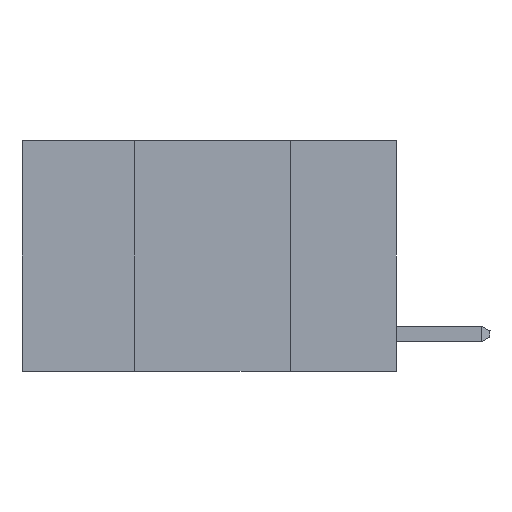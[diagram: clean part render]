
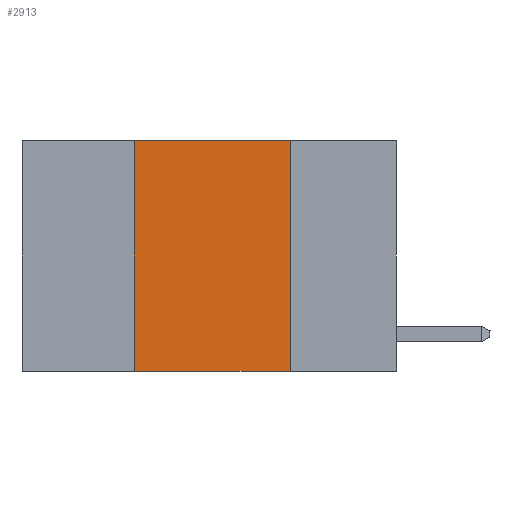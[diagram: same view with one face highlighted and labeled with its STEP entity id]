
A CAD part, left-side view. The second image highlights one B-rep face of the part: STEP entity #2913.
In plain terms, the highlighted planar face has unit normal (-1, 0, 0).
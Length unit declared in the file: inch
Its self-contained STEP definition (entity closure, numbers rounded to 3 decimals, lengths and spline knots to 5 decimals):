
#438 = CARTESIAN_POINT ( 'NONE',  ( 0., 0.17, 0. ) ) ;
#893 = VECTOR ( 'NONE', #7724, 39.37008 ) ;
#957 = LINE ( 'NONE', #9798, #1074 ) ;
#1074 = VECTOR ( 'NONE', #5204, 39.37008 ) ;
#2290 = DIRECTION ( 'NONE',  ( 0., -1., 0. ) ) ;
#2453 = CARTESIAN_POINT ( 'NONE',  ( 0., 0.17, 0. ) ) ;
#2671 = CARTESIAN_POINT ( 'NONE',  ( 0., 0.6, -0.37 ) ) ;
#2913 = ADVANCED_FACE ( 'NONE', ( #14982 ), #18160, .F. ) ;
#2950 = ORIENTED_EDGE ( 'NONE', *, *, #8047, .F. ) ;
#4691 = AXIS2_PLACEMENT_3D ( 'NONE', #7805, #10606, #16529 ) ;
#5204 = DIRECTION ( 'NONE',  ( 0., 0., 1. ) ) ;
#6109 = EDGE_LOOP ( 'NONE', ( #2950, #14230, #10822, #17636 ) ) ;
#6267 = CARTESIAN_POINT ( 'NONE',  ( 0., 0.42, 0. ) ) ;
#6475 = VERTEX_POINT ( 'NONE', #2453 ) ;
#7020 = EDGE_CURVE ( 'NONE', #18654, #6475, #7302, .T. ) ;
#7302 = LINE ( 'NONE', #9135, #10634 ) ;
#7724 = DIRECTION ( 'NONE',  ( 0., 0., -1. ) ) ;
#7805 = CARTESIAN_POINT ( 'NONE',  ( 0., 0.6, 0. ) ) ;
#8047 = EDGE_CURVE ( 'NONE', #6475, #12173, #13732, .T. ) ;
#9135 = CARTESIAN_POINT ( 'NONE',  ( 0., 0.6, 0. ) ) ;
#9798 = CARTESIAN_POINT ( 'NONE',  ( 0., 0.42, 0. ) ) ;
#10606 = DIRECTION ( 'NONE',  ( 1., 0., 0. ) ) ;
#10634 = VECTOR ( 'NONE', #14945, 39.37008 ) ;
#10822 = ORIENTED_EDGE ( 'NONE', *, *, #12796, .F. ) ;
#12173 = VERTEX_POINT ( 'NONE', #17082 ) ;
#12796 = EDGE_CURVE ( 'NONE', #15802, #18654, #957, .T. ) ;
#13732 = LINE ( 'NONE', #438, #893 ) ;
#14230 = ORIENTED_EDGE ( 'NONE', *, *, #7020, .F. ) ;
#14513 = VECTOR ( 'NONE', #2290, 39.37008 ) ;
#14945 = DIRECTION ( 'NONE',  ( 0., -1., 0. ) ) ;
#14982 = FACE_OUTER_BOUND ( 'NONE', #6109, .T. ) ;
#15041 = CARTESIAN_POINT ( 'NONE',  ( 0., 0.42, -0.37 ) ) ;
#15802 = VERTEX_POINT ( 'NONE', #15041 ) ;
#16529 = DIRECTION ( 'NONE',  ( 0., 0., -1. ) ) ;
#17082 = CARTESIAN_POINT ( 'NONE',  ( 0., 0.17, -0.37 ) ) ;
#17429 = LINE ( 'NONE', #2671, #14513 ) ;
#17636 = ORIENTED_EDGE ( 'NONE', *, *, #18460, .T. ) ;
#18160 = PLANE ( 'NONE',  #4691 ) ;
#18460 = EDGE_CURVE ( 'NONE', #15802, #12173, #17429, .T. ) ;
#18654 = VERTEX_POINT ( 'NONE', #6267 ) ;
